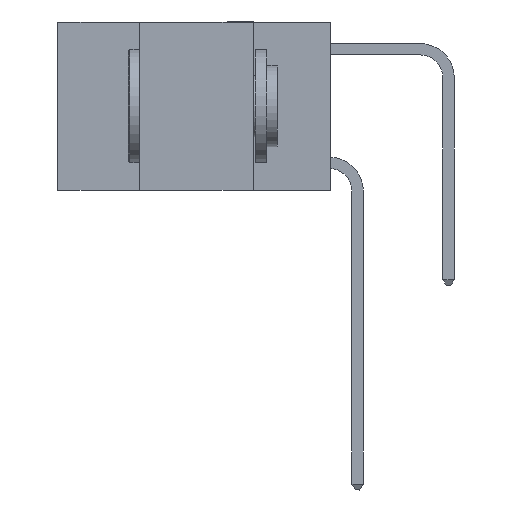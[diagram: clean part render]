
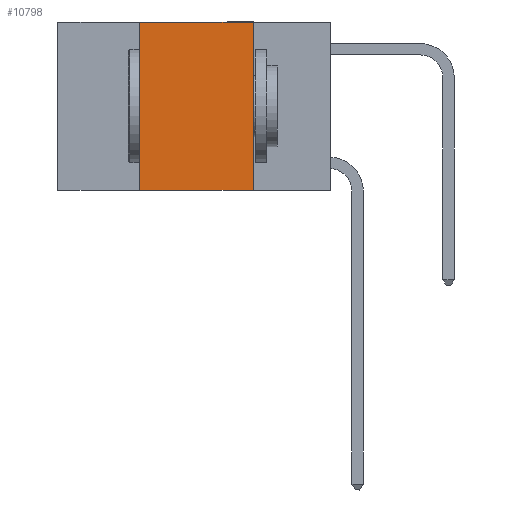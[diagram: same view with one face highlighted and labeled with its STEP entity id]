
A CAD part, left-side view. The second image highlights one B-rep face of the part: STEP entity #10798.
In plain terms, the highlighted planar face has unit normal (-1, 0, 0).
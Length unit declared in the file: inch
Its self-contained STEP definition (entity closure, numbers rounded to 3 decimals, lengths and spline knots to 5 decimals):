
#63 = PLANE ( 'NONE',  #11037 ) ;
#153 = EDGE_CURVE ( 'NONE', #10585, #11876, #11678, .T. ) ;
#973 = CARTESIAN_POINT ( 'NONE',  ( 0., 0.17, 0. ) ) ;
#1276 = FACE_OUTER_BOUND ( 'NONE', #2392, .T. ) ;
#1401 = DIRECTION ( 'NONE',  ( 0., 0., -1. ) ) ;
#2392 = EDGE_LOOP ( 'NONE', ( #8850, #2538, #3463, #6175 ) ) ;
#2538 = ORIENTED_EDGE ( 'NONE', *, *, #4200, .F. ) ;
#2855 = VECTOR ( 'NONE', #1401, 39.37008 ) ;
#2904 = CARTESIAN_POINT ( 'NONE',  ( 0., 0.17, -0.37 ) ) ;
#3463 = ORIENTED_EDGE ( 'NONE', *, *, #11782, .F. ) ;
#3691 = CARTESIAN_POINT ( 'NONE',  ( 0., 0.6, 0. ) ) ;
#3854 = CARTESIAN_POINT ( 'NONE',  ( 0., 0.42, 0. ) ) ;
#4065 = LINE ( 'NONE', #11825, #12468 ) ;
#4200 = EDGE_CURVE ( 'NONE', #6736, #10585, #7712, .T. ) ;
#4725 = CARTESIAN_POINT ( 'NONE',  ( 0., 0.17, 0. ) ) ;
#4805 = VECTOR ( 'NONE', #13132, 39.37008 ) ;
#5909 = VERTEX_POINT ( 'NONE', #12508 ) ;
#5986 = DIRECTION ( 'NONE',  ( 1., 0., 0. ) ) ;
#6175 = ORIENTED_EDGE ( 'NONE', *, *, #10316, .T. ) ;
#6736 = VERTEX_POINT ( 'NONE', #3854 ) ;
#7295 = CARTESIAN_POINT ( 'NONE',  ( 0., 0.42, 0. ) ) ;
#7338 = LINE ( 'NONE', #7295, #10205 ) ;
#7712 = LINE ( 'NONE', #13089, #4805 ) ;
#8390 = DIRECTION ( 'NONE',  ( 0., 0., 1. ) ) ;
#8850 = ORIENTED_EDGE ( 'NONE', *, *, #153, .F. ) ;
#10205 = VECTOR ( 'NONE', #8390, 39.37008 ) ;
#10316 = EDGE_CURVE ( 'NONE', #5909, #11876, #4065, .T. ) ;
#10585 = VERTEX_POINT ( 'NONE', #973 ) ;
#10798 = ADVANCED_FACE ( 'NONE', ( #1276 ), #63, .F. ) ;
#11037 = AXIS2_PLACEMENT_3D ( 'NONE', #3691, #5986, #13543 ) ;
#11678 = LINE ( 'NONE', #4725, #2855 ) ;
#11782 = EDGE_CURVE ( 'NONE', #5909, #6736, #7338, .T. ) ;
#11825 = CARTESIAN_POINT ( 'NONE',  ( 0., 0.6, -0.37 ) ) ;
#11876 = VERTEX_POINT ( 'NONE', #2904 ) ;
#12468 = VECTOR ( 'NONE', #12916, 39.37008 ) ;
#12508 = CARTESIAN_POINT ( 'NONE',  ( 0., 0.42, -0.37 ) ) ;
#12916 = DIRECTION ( 'NONE',  ( 0., -1., 0. ) ) ;
#13089 = CARTESIAN_POINT ( 'NONE',  ( 0., 0.6, 0. ) ) ;
#13132 = DIRECTION ( 'NONE',  ( 0., -1., 0. ) ) ;
#13543 = DIRECTION ( 'NONE',  ( 0., 0., -1. ) ) ;
